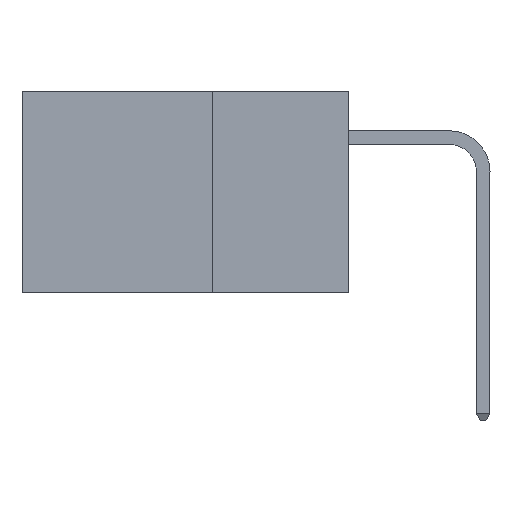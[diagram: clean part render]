
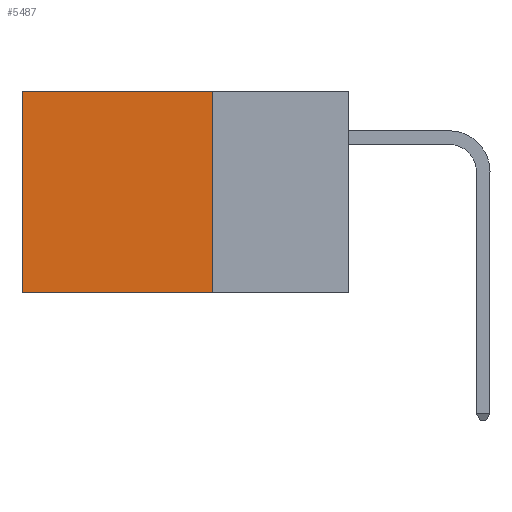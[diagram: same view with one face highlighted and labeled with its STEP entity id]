
A CAD part, left-side view. The second image highlights one B-rep face of the part: STEP entity #5487.
In plain terms, the highlighted planar face has unit normal (-1, 0, 0).
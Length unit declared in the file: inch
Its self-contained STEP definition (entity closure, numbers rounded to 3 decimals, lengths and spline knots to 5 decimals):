
#542 = EDGE_CURVE ( 'NONE', #15947, #15645, #4019, .T. ) ;
#640 = VECTOR ( 'NONE', #1910, 39.37008 ) ;
#815 = EDGE_CURVE ( 'NONE', #14233, #1679, #3017, .T. ) ;
#1145 = DIRECTION ( 'NONE',  ( 0., 1., 0. ) ) ;
#1679 = VERTEX_POINT ( 'NONE', #3591 ) ;
#1742 = CARTESIAN_POINT ( 'NONE',  ( 0.2875, 0.25, 0. ) ) ;
#1910 = DIRECTION ( 'NONE',  ( 0., 1., 0. ) ) ;
#3017 = LINE ( 'NONE', #16109, #12595 ) ;
#3463 = DIRECTION ( 'NONE',  ( 0., 0., -1. ) ) ;
#3591 = CARTESIAN_POINT ( 'NONE',  ( 0.2875, 0.6, -0.37 ) ) ;
#3672 = ORIENTED_EDGE ( 'NONE', *, *, #9983, .T. ) ;
#4019 = LINE ( 'NONE', #8185, #640 ) ;
#4094 = DIRECTION ( 'NONE',  ( 1., 0., 0. ) ) ;
#5487 = ADVANCED_FACE ( 'NONE', ( #11601 ), #11617, .F. ) ;
#6141 = EDGE_CURVE ( 'NONE', #15947, #14233, #8848, .T. ) ;
#6188 = EDGE_LOOP ( 'NONE', ( #3672, #12727, #7019, #14444 ) ) ;
#6675 = DIRECTION ( 'NONE',  ( 0., 0., -1. ) ) ;
#7019 = ORIENTED_EDGE ( 'NONE', *, *, #6141, .F. ) ;
#8077 = DIRECTION ( 'NONE',  ( 0., 0., -1. ) ) ;
#8185 = CARTESIAN_POINT ( 'NONE',  ( 0.2875, 0.25, 0. ) ) ;
#8848 = LINE ( 'NONE', #1742, #15074 ) ;
#9983 = EDGE_CURVE ( 'NONE', #15645, #1679, #15550, .T. ) ;
#10401 = AXIS2_PLACEMENT_3D ( 'NONE', #12865, #4094, #6675 ) ;
#11516 = CARTESIAN_POINT ( 'NONE',  ( 0.2875, 0.6, 0. ) ) ;
#11601 = FACE_OUTER_BOUND ( 'NONE', #6188, .T. ) ;
#11617 = PLANE ( 'NONE',  #10401 ) ;
#12073 = CARTESIAN_POINT ( 'NONE',  ( 0.2875, 0.25, -0.37 ) ) ;
#12199 = CARTESIAN_POINT ( 'NONE',  ( 0.2875, 0.6, 0. ) ) ;
#12595 = VECTOR ( 'NONE', #1145, 39.37008 ) ;
#12647 = VECTOR ( 'NONE', #3463, 39.37008 ) ;
#12727 = ORIENTED_EDGE ( 'NONE', *, *, #815, .F. ) ;
#12865 = CARTESIAN_POINT ( 'NONE',  ( 0.2875, 0.25, 0. ) ) ;
#14233 = VERTEX_POINT ( 'NONE', #12073 ) ;
#14444 = ORIENTED_EDGE ( 'NONE', *, *, #542, .T. ) ;
#15074 = VECTOR ( 'NONE', #8077, 39.37008 ) ;
#15550 = LINE ( 'NONE', #12199, #12647 ) ;
#15645 = VERTEX_POINT ( 'NONE', #11516 ) ;
#15725 = CARTESIAN_POINT ( 'NONE',  ( 0.2875, 0.25, 0. ) ) ;
#15947 = VERTEX_POINT ( 'NONE', #15725 ) ;
#16109 = CARTESIAN_POINT ( 'NONE',  ( 0.2875, 0.25, -0.37 ) ) ;
